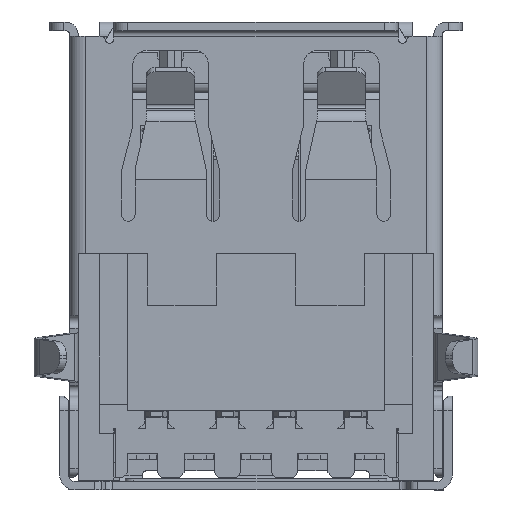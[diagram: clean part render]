
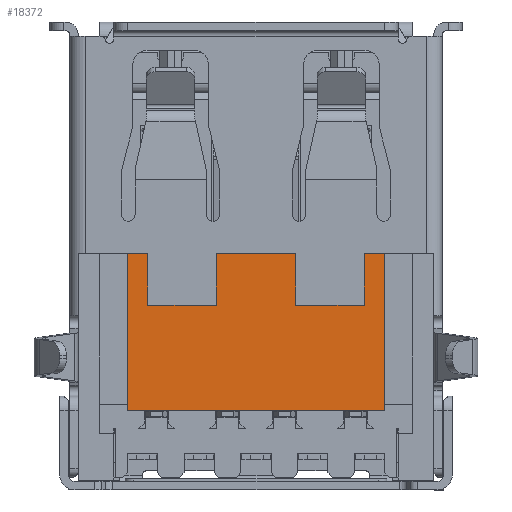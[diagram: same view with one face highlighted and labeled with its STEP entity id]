
A CAD part, front view. The second image highlights one B-rep face of the part: STEP entity #18372.
In plain terms, the highlighted face is planar.
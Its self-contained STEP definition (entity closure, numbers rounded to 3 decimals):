
#767 = DIRECTION ( 'NONE',  ( 0., 1., 0. ) ) ;
#1698 = LINE ( 'NONE', #14021, #19263 ) ;
#1844 = VECTOR ( 'NONE', #33764, 1000. ) ;
#3799 = FACE_OUTER_BOUND ( 'NONE', #74378, .T. ) ;
#4278 = ORIENTED_EDGE ( 'NONE', *, *, #45015, .T. ) ;
#4772 = ORIENTED_EDGE ( 'NONE', *, *, #55942, .T. ) ;
#5178 = EDGE_CURVE ( 'NONE', #62614, #73437, #31093, .T. ) ;
#6119 = ORIENTED_EDGE ( 'NONE', *, *, #15264, .T. ) ;
#7370 = VECTOR ( 'NONE', #45004, 1000. ) ;
#8742 = CARTESIAN_POINT ( 'NONE',  ( 0., -2.33, 4.13 ) ) ;
#9091 = VERTEX_POINT ( 'NONE', #9540 ) ;
#9222 = VERTEX_POINT ( 'NONE', #17065 ) ;
#9340 = DIRECTION ( 'NONE',  ( -1., 0., 0. ) ) ;
#9540 = CARTESIAN_POINT ( 'NONE',  ( 4.5, 3.17, 4.13 ) ) ;
#9888 = CARTESIAN_POINT ( 'NONE',  ( -4.5, -2.33, 4.13 ) ) ;
#11107 = DIRECTION ( 'NONE',  ( 0., -1., 0. ) ) ;
#11132 = EDGE_CURVE ( 'NONE', #47342, #20844, #53100, .T. ) ;
#11336 = DIRECTION ( 'NONE',  ( 1., 0., 0. ) ) ;
#11693 = LINE ( 'NONE', #78181, #28786 ) ;
#12277 = VERTEX_POINT ( 'NONE', #28514 ) ;
#14021 = CARTESIAN_POINT ( 'NONE',  ( -6.225, -2.33, 4.13 ) ) ;
#15264 = EDGE_CURVE ( 'NONE', #20844, #12277, #11693, .T. ) ;
#16501 = EDGE_CURVE ( 'NONE', #73437, #51140, #77198, .T. ) ;
#16697 = ORIENTED_EDGE ( 'NONE', *, *, #50207, .F. ) ;
#17065 = CARTESIAN_POINT ( 'NONE',  ( 4.5, -2.33, 4.13 ) ) ;
#17243 = VERTEX_POINT ( 'NONE', #33207 ) ;
#17687 = PLANE ( 'NONE',  #20052 ) ;
#17974 = VECTOR ( 'NONE', #22128, 1000. ) ;
#18372 = ADVANCED_FACE ( 'NONE', ( #3799 ), #17687, .T. ) ;
#18801 = CARTESIAN_POINT ( 'NONE',  ( -6.225, -2.33, 4.13 ) ) ;
#19002 = VECTOR ( 'NONE', #767, 1000. ) ;
#19183 = LINE ( 'NONE', #18801, #58949 ) ;
#19263 = VECTOR ( 'NONE', #37872, 1000. ) ;
#20052 = AXIS2_PLACEMENT_3D ( 'NONE', #23658, #34009, #11336 ) ;
#20844 = VERTEX_POINT ( 'NONE', #22793 ) ;
#22128 = DIRECTION ( 'NONE',  ( 0., -1., 0. ) ) ;
#22229 = VECTOR ( 'NONE', #9340, 1000. ) ;
#22270 = VERTEX_POINT ( 'NONE', #67281 ) ;
#22793 = CARTESIAN_POINT ( 'NONE',  ( 3.8, -0.53, 4.13 ) ) ;
#23658 = CARTESIAN_POINT ( 'NONE',  ( 0., 5.62, 4.13 ) ) ;
#26103 = EDGE_CURVE ( 'NONE', #17243, #62614, #43824, .T. ) ;
#27215 = LINE ( 'NONE', #39127, #43941 ) ;
#28008 = LINE ( 'NONE', #77777, #22229 ) ;
#28514 = CARTESIAN_POINT ( 'NONE',  ( 3.8, -2.33, 4.13 ) ) ;
#28786 = VECTOR ( 'NONE', #48672, 1000. ) ;
#28809 = DIRECTION ( 'NONE',  ( 1., 0., 0. ) ) ;
#29804 = ORIENTED_EDGE ( 'NONE', *, *, #77558, .T. ) ;
#29821 = LINE ( 'NONE', #66053, #19002 ) ;
#31093 = LINE ( 'NONE', #73722, #68158 ) ;
#31399 = VECTOR ( 'NONE', #11107, 1000. ) ;
#32727 = ORIENTED_EDGE ( 'NONE', *, *, #43609, .T. ) ;
#33207 = CARTESIAN_POINT ( 'NONE',  ( -3.8, -2.33, 4.13 ) ) ;
#33764 = DIRECTION ( 'NONE',  ( 1., 0., 0. ) ) ;
#34009 = DIRECTION ( 'NONE',  ( 0., 0., 1. ) ) ;
#34047 = CARTESIAN_POINT ( 'NONE',  ( -4.5, 5.62, 4.13 ) ) ;
#37713 = ORIENTED_EDGE ( 'NONE', *, *, #11132, .T. ) ;
#37829 = DIRECTION ( 'NONE',  ( 1., 0., 0. ) ) ;
#37834 = CARTESIAN_POINT ( 'NONE',  ( -3.8, 5.62, 4.13 ) ) ;
#37872 = DIRECTION ( 'NONE',  ( -1., 0., 0. ) ) ;
#39127 = CARTESIAN_POINT ( 'NONE',  ( 4.5, 5.62, 4.13 ) ) ;
#41822 = CARTESIAN_POINT ( 'NONE',  ( 1.4, -0.53, 4.13 ) ) ;
#41839 = ORIENTED_EDGE ( 'NONE', *, *, #52691, .F. ) ;
#43609 = EDGE_CURVE ( 'NONE', #9091, #60530, #28008, .T. ) ;
#43824 = LINE ( 'NONE', #37834, #7370 ) ;
#43941 = VECTOR ( 'NONE', #51888, 1000. ) ;
#45004 = DIRECTION ( 'NONE',  ( 0., 1., 0. ) ) ;
#45015 = EDGE_CURVE ( 'NONE', #51140, #22270, #64419, .T. ) ;
#46913 = ORIENTED_EDGE ( 'NONE', *, *, #26103, .T. ) ;
#47342 = VERTEX_POINT ( 'NONE', #41822 ) ;
#48213 = CARTESIAN_POINT ( 'NONE',  ( -4.5, 3.17, 4.13 ) ) ;
#48672 = DIRECTION ( 'NONE',  ( 0., -1., 0. ) ) ;
#50207 = EDGE_CURVE ( 'NONE', #9222, #12277, #1698, .T. ) ;
#51140 = VERTEX_POINT ( 'NONE', #78173 ) ;
#51888 = DIRECTION ( 'NONE',  ( 0., 1., 0. ) ) ;
#52317 = CARTESIAN_POINT ( 'NONE',  ( 3.8, -0.53, 4.13 ) ) ;
#52672 = CARTESIAN_POINT ( 'NONE',  ( -1.4, -0.53, 4.13 ) ) ;
#52691 = EDGE_CURVE ( 'NONE', #17243, #72569, #19183, .T. ) ;
#53100 = LINE ( 'NONE', #52317, #59234 ) ;
#55942 = EDGE_CURVE ( 'NONE', #9222, #9091, #27215, .T. ) ;
#57935 = CARTESIAN_POINT ( 'NONE',  ( -3.8, -0.53, 4.13 ) ) ;
#58949 = VECTOR ( 'NONE', #65785, 1000. ) ;
#59234 = VECTOR ( 'NONE', #28809, 1000. ) ;
#59816 = ORIENTED_EDGE ( 'NONE', *, *, #16501, .T. ) ;
#60530 = VERTEX_POINT ( 'NONE', #48213 ) ;
#62614 = VERTEX_POINT ( 'NONE', #57935 ) ;
#64419 = LINE ( 'NONE', #8742, #1844 ) ;
#64799 = ORIENTED_EDGE ( 'NONE', *, *, #67652, .T. ) ;
#65252 = CARTESIAN_POINT ( 'NONE',  ( -1.4, 5.62, 4.13 ) ) ;
#65511 = LINE ( 'NONE', #34047, #17974 ) ;
#65785 = DIRECTION ( 'NONE',  ( -1., 0., 0. ) ) ;
#66053 = CARTESIAN_POINT ( 'NONE',  ( 1.4, 5.62, 4.13 ) ) ;
#67281 = CARTESIAN_POINT ( 'NONE',  ( 1.4, -2.33, 4.13 ) ) ;
#67652 = EDGE_CURVE ( 'NONE', #22270, #47342, #29821, .T. ) ;
#68158 = VECTOR ( 'NONE', #37829, 1000. ) ;
#69333 = ORIENTED_EDGE ( 'NONE', *, *, #5178, .T. ) ;
#72569 = VERTEX_POINT ( 'NONE', #9888 ) ;
#73437 = VERTEX_POINT ( 'NONE', #52672 ) ;
#73722 = CARTESIAN_POINT ( 'NONE',  ( -1.4, -0.53, 4.13 ) ) ;
#74378 = EDGE_LOOP ( 'NONE', ( #29804, #41839, #46913, #69333, #59816, #4278, #64799, #37713, #6119, #16697, #4772, #32727 ) ) ;
#77198 = LINE ( 'NONE', #65252, #31399 ) ;
#77558 = EDGE_CURVE ( 'NONE', #60530, #72569, #65511, .T. ) ;
#77777 = CARTESIAN_POINT ( 'NONE',  ( 0., 3.17, 4.13 ) ) ;
#78173 = CARTESIAN_POINT ( 'NONE',  ( -1.4, -2.33, 4.13 ) ) ;
#78181 = CARTESIAN_POINT ( 'NONE',  ( 3.8, 5.62, 4.13 ) ) ;
